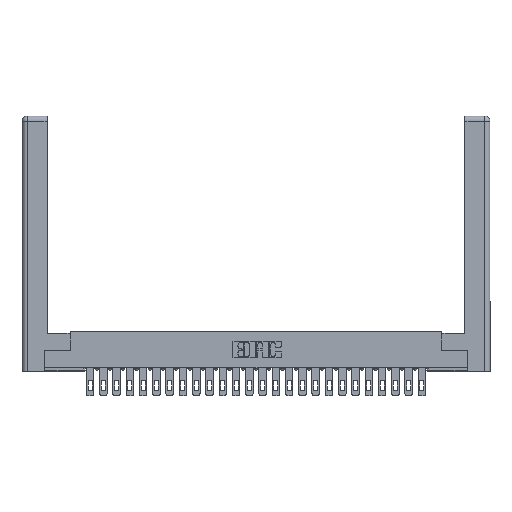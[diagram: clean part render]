
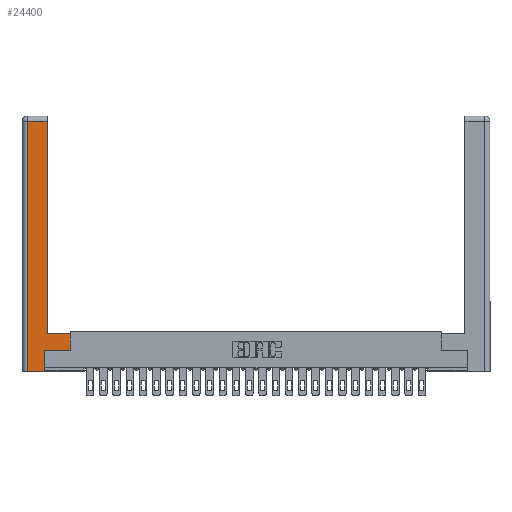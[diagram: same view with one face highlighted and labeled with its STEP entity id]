
A CAD part, top view. The second image highlights one B-rep face of the part: STEP entity #24400.
In plain terms, the highlighted planar face has unit normal (0, 0, 1).
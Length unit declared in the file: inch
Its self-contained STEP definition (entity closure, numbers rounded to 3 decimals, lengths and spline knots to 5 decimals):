
#415 = CARTESIAN_POINT ( 'NONE',  ( 0.295, 0.45, 0. ) ) ;
#537 = DIRECTION ( 'NONE',  ( 1., 0., 0. ) ) ;
#552 = VERTEX_POINT ( 'NONE', #415 ) ;
#1497 = ORIENTED_EDGE ( 'NONE', *, *, #9801, .T. ) ;
#1998 = AXIS2_PLACEMENT_3D ( 'NONE', #4099, #27572, #18998 ) ;
#2165 = CARTESIAN_POINT ( 'NONE',  ( 0.295, 3., 0. ) ) ;
#3076 = EDGE_LOOP ( 'NONE', ( #15441, #5603, #26133, #11608, #13182, #1497, #4683, #17539 ) ) ;
#3297 = EDGE_CURVE ( 'NONE', #25731, #18924, #21639, .T. ) ;
#3680 = EDGE_CURVE ( 'NONE', #21832, #10214, #22634, .T. ) ;
#4071 = VECTOR ( 'NONE', #537, 39.37008 ) ;
#4099 = CARTESIAN_POINT ( 'NONE',  ( 0., 0., 0. ) ) ;
#4683 = ORIENTED_EDGE ( 'NONE', *, *, #25501, .T. ) ;
#4923 = VERTEX_POINT ( 'NONE', #5949 ) ;
#5195 = VECTOR ( 'NONE', #27695, 39.37008 ) ;
#5473 = LINE ( 'NONE', #2165, #26865 ) ;
#5603 = ORIENTED_EDGE ( 'NONE', *, *, #3680, .T. ) ;
#5949 = CARTESIAN_POINT ( 'NONE',  ( 0.0615, 0., 0. ) ) ;
#6196 = DIRECTION ( 'NONE',  ( -1., 0., 0. ) ) ;
#7174 = LINE ( 'NONE', #22671, #19892 ) ;
#8000 = CARTESIAN_POINT ( 'NONE',  ( 0.565, 0.45, 0. ) ) ;
#8957 = CARTESIAN_POINT ( 'NONE',  ( 0.265, 0.245, 0. ) ) ;
#9752 = CARTESIAN_POINT ( 'NONE',  ( 0.565, 0.45, 0. ) ) ;
#9801 = EDGE_CURVE ( 'NONE', #18924, #13056, #24581, .T. ) ;
#10214 = VERTEX_POINT ( 'NONE', #25347 ) ;
#10348 = DIRECTION ( 'NONE',  ( 0., 1., 0. ) ) ;
#10396 = PLANE ( 'NONE',  #1998 ) ;
#11153 = CARTESIAN_POINT ( 'NONE',  ( 0.265, 0., 0. ) ) ;
#11277 = VECTOR ( 'NONE', #6196, 39.37008 ) ;
#11608 = ORIENTED_EDGE ( 'NONE', *, *, #21351, .T. ) ;
#12016 = DIRECTION ( 'NONE',  ( -1., 0., 0. ) ) ;
#12807 = EDGE_CURVE ( 'NONE', #14503, #552, #19136, .T. ) ;
#13056 = VERTEX_POINT ( 'NONE', #18739 ) ;
#13071 = CARTESIAN_POINT ( 'NONE',  ( 0.265, 0.245, 0. ) ) ;
#13182 = ORIENTED_EDGE ( 'NONE', *, *, #3297, .T. ) ;
#13324 = DIRECTION ( 'NONE',  ( 0., 1., 0. ) ) ;
#13439 = VECTOR ( 'NONE', #12016, 39.37008 ) ;
#14142 = DIRECTION ( 'NONE',  ( 0., 1., 0. ) ) ;
#14503 = VERTEX_POINT ( 'NONE', #9752 ) ;
#14780 = CARTESIAN_POINT ( 'NONE',  ( 0.265, 0., 0. ) ) ;
#15441 = ORIENTED_EDGE ( 'NONE', *, *, #20694, .T. ) ;
#16023 = CARTESIAN_POINT ( 'NONE',  ( 0.295, 0.45, 0. ) ) ;
#16644 = CARTESIAN_POINT ( 'NONE',  ( 0.295, 2.94, 0. ) ) ;
#17539 = ORIENTED_EDGE ( 'NONE', *, *, #12807, .T. ) ;
#18541 = CARTESIAN_POINT ( 'NONE',  ( 0.0615, 2.94, 0. ) ) ;
#18739 = CARTESIAN_POINT ( 'NONE',  ( 0.565, 0.245, 0. ) ) ;
#18924 = VERTEX_POINT ( 'NONE', #13071 ) ;
#18998 = DIRECTION ( 'NONE',  ( -1., 0., 0. ) ) ;
#19136 = LINE ( 'NONE', #16023, #13439 ) ;
#19677 = EDGE_CURVE ( 'NONE', #10214, #4923, #7174, .T. ) ;
#19892 = VECTOR ( 'NONE', #20511, 39.37008 ) ;
#20511 = DIRECTION ( 'NONE',  ( 0., -1., 0. ) ) ;
#20694 = EDGE_CURVE ( 'NONE', #552, #21832, #5473, .T. ) ;
#21351 = EDGE_CURVE ( 'NONE', #4923, #25731, #26812, .T. ) ;
#21639 = LINE ( 'NONE', #8957, #24324 ) ;
#21832 = VERTEX_POINT ( 'NONE', #16644 ) ;
#22634 = LINE ( 'NONE', #18541, #11277 ) ;
#22671 = CARTESIAN_POINT ( 'NONE',  ( 0.0615, 0., 0. ) ) ;
#22994 = FACE_OUTER_BOUND ( 'NONE', #3076, .T. ) ;
#24324 = VECTOR ( 'NONE', #13324, 39.37008 ) ;
#24400 = ADVANCED_FACE ( 'NONE', ( #22994 ), #10396, .F. ) ;
#24559 = LINE ( 'NONE', #8000, #27243 ) ;
#24581 = LINE ( 'NONE', #25551, #5195 ) ;
#25347 = CARTESIAN_POINT ( 'NONE',  ( 0.0615, 2.94, 0. ) ) ;
#25501 = EDGE_CURVE ( 'NONE', #13056, #14503, #24559, .T. ) ;
#25551 = CARTESIAN_POINT ( 'NONE',  ( 0.565, 0.245, 0. ) ) ;
#25731 = VERTEX_POINT ( 'NONE', #14780 ) ;
#26133 = ORIENTED_EDGE ( 'NONE', *, *, #19677, .T. ) ;
#26812 = LINE ( 'NONE', #11153, #4071 ) ;
#26865 = VECTOR ( 'NONE', #10348, 39.37008 ) ;
#27243 = VECTOR ( 'NONE', #14142, 39.37008 ) ;
#27572 = DIRECTION ( 'NONE',  ( 0., 0., -1. ) ) ;
#27695 = DIRECTION ( 'NONE',  ( 1., 0., 0. ) ) ;
